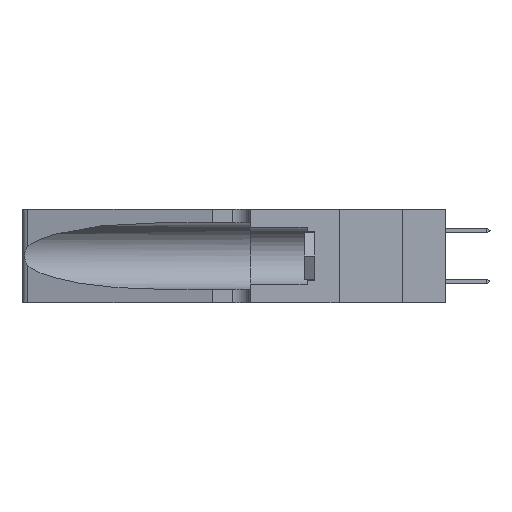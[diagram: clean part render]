
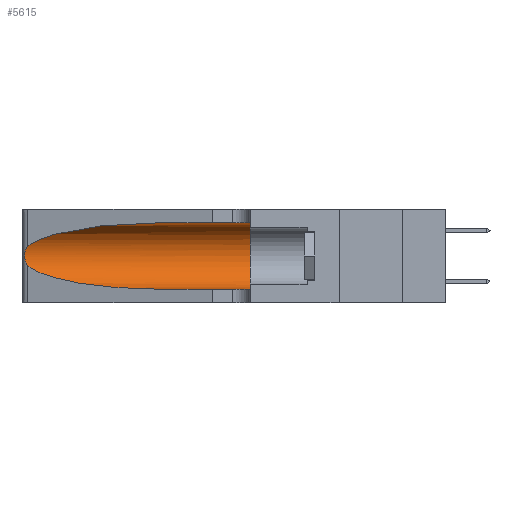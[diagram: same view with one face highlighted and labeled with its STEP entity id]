
A CAD part, left-side view. The second image highlights one B-rep face of the part: STEP entity #5615.
In plain terms, the highlighted cylindrical face has radius 3.308 mm (diameter 6.617 mm), a partial arc.
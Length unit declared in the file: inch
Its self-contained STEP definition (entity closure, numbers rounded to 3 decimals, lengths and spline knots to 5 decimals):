
#979 =( BOUNDED_CURVE ( )  B_SPLINE_CURVE ( 3, ( #26609, #16413, #6834, #9188 ),
 .UNSPECIFIED., .F., .F. ) 
 B_SPLINE_CURVE_WITH_KNOTS ( ( 4, 4 ),
 ( 3.44316, 4.71239 ),
 .UNSPECIFIED. ) 
 CURVE ( )  GEOMETRIC_REPRESENTATION_ITEM ( )  RATIONAL_B_SPLINE_CURVE ( ( 1., 0.87, 0.87, 1. ) ) 
 REPRESENTATION_ITEM ( '' )  );
#1558 = VECTOR ( 'NONE', #3697, 39.37008 ) ;
#1988 = CARTESIAN_POINT ( 'NONE',  ( 0.1305, 0.72297, 0.31525 ) ) ;
#2297 = CARTESIAN_POINT ( 'NONE',  ( 0.25854, 1.2359, 0.20912 ) ) ;
#2803 = DIRECTION ( 'NONE',  ( 0., 0., 1. ) ) ;
#3655 = DIRECTION ( 'NONE',  ( 0., -1., 0. ) ) ;
#3697 = DIRECTION ( 'NONE',  ( 0., -1., 0. ) ) ;
#3764 = CARTESIAN_POINT ( 'NONE',  ( 0.25487, 1.22718, 0.14631 ) ) ;
#3884 = CARTESIAN_POINT ( 'NONE',  ( 0.1305, 1.61858, 0.31525 ) ) ;
#3975 =( BOUNDED_CURVE ( )  B_SPLINE_CURVE ( 3, ( #1988, #10288, #7397, #22327 ),
 .UNSPECIFIED., .F., .F. ) 
 B_SPLINE_CURVE_WITH_KNOTS ( ( 4, 4 ),
 ( 1.5708, 2.84003 ),
 .UNSPECIFIED. ) 
 CURVE ( )  GEOMETRIC_REPRESENTATION_ITEM ( )  RATIONAL_B_SPLINE_CURVE ( ( 1., 0.87, 0.87, 1. ) ) 
 REPRESENTATION_ITEM ( '' )  );
#4960 = EDGE_LOOP ( 'NONE', ( #15871, #28062, #21930, #26043, #31861, #14223 ) ) ;
#5230 = CARTESIAN_POINT ( 'NONE',  ( 0.25555, 1.22994, 0.2215 ) ) ;
#5615 = ADVANCED_FACE ( 'NONE', ( #18516 ), #10312, .F. ) ;
#5752 = B_SPLINE_CURVE_WITH_KNOTS ( 'NONE', 3,
 ( #9812, #5230, #18778, #13718, #2297, #28128, #29218, #25116, #11367, #16206, #8639, #28773, #31271, #3764 ),
 .UNSPECIFIED., .F., .F.,
 ( 4, 2, 2, 2, 2, 2, 4 ),
 ( 0., 0.00027, 0.00053, 0.00107, 0.0016, 0.00187, 0.00214 ),
 .UNSPECIFIED. ) ;
#6315 = AXIS2_PLACEMENT_3D ( 'NONE', #17708, #27797, #2803 ) ;
#6834 = CARTESIAN_POINT ( 'NONE',  ( 0.18966, 0.96281, 0.05475 ) ) ;
#7397 = CARTESIAN_POINT ( 'NONE',  ( 0.2373, 1.15595, 0.28018 ) ) ;
#8072 = CIRCLE ( 'NONE', #6315, 0.13025 ) ;
#8535 = VERTEX_POINT ( 'NONE', #23528 ) ;
#8639 = CARTESIAN_POINT ( 'NONE',  ( 0.25789, 1.23486, 0.15765 ) ) ;
#8794 = CARTESIAN_POINT ( 'NONE',  ( 0.1305, 1.61858, 0.05475 ) ) ;
#9188 = CARTESIAN_POINT ( 'NONE',  ( 0.1305, 0.72297, 0.05475 ) ) ;
#9275 = CARTESIAN_POINT ( 'NONE',  ( 0.1305, 1.61858, 0.185 ) ) ;
#9812 = CARTESIAN_POINT ( 'NONE',  ( 0.25487, 1.22718, 0.22369 ) ) ;
#10288 = CARTESIAN_POINT ( 'NONE',  ( 0.18966, 0.96281, 0.31525 ) ) ;
#10312 = CYLINDRICAL_SURFACE ( 'NONE', #31719, 0.13025 ) ;
#10435 = EDGE_CURVE ( 'NONE', #23699, #16093, #979, .T. ) ;
#11166 = CARTESIAN_POINT ( 'NONE',  ( 0.1305, 0.35, 0.31525 ) ) ;
#11367 = CARTESIAN_POINT ( 'NONE',  ( 0.26017, 1.23833, 0.17102 ) ) ;
#11415 = CARTESIAN_POINT ( 'NONE',  ( 0.25487, 1.22718, 0.22369 ) ) ;
#13718 = CARTESIAN_POINT ( 'NONE',  ( 0.25787, 1.23484, 0.2124 ) ) ;
#14040 = EDGE_CURVE ( 'NONE', #26990, #23699, #5752, .T. ) ;
#14223 = ORIENTED_EDGE ( 'NONE', *, *, #25678, .F. ) ;
#15762 = CARTESIAN_POINT ( 'NONE',  ( 0.1305, 0.72297, 0.05475 ) ) ;
#15871 = ORIENTED_EDGE ( 'NONE', *, *, #27220, .T. ) ;
#16093 = VERTEX_POINT ( 'NONE', #15762 ) ;
#16206 = CARTESIAN_POINT ( 'NONE',  ( 0.25856, 1.23593, 0.16098 ) ) ;
#16413 = CARTESIAN_POINT ( 'NONE',  ( 0.2373, 1.15595, 0.08982 ) ) ;
#16650 = VERTEX_POINT ( 'NONE', #24697 ) ;
#17708 = CARTESIAN_POINT ( 'NONE',  ( 0.1305, 0.35, 0.185 ) ) ;
#18516 = FACE_OUTER_BOUND ( 'NONE', #4960, .T. ) ;
#18778 = CARTESIAN_POINT ( 'NONE',  ( 0.25639, 1.23184, 0.21858 ) ) ;
#19902 = LINE ( 'NONE', #3884, #31514 ) ;
#21930 = ORIENTED_EDGE ( 'NONE', *, *, #10435, .T. ) ;
#22327 = CARTESIAN_POINT ( 'NONE',  ( 0.25487, 1.22718, 0.22369 ) ) ;
#23528 = CARTESIAN_POINT ( 'NONE',  ( 0.1305, 0.35, 0.05475 ) ) ;
#23699 = VERTEX_POINT ( 'NONE', #31519 ) ;
#24697 = CARTESIAN_POINT ( 'NONE',  ( 0.1305, 0.72297, 0.31525 ) ) ;
#24858 = LINE ( 'NONE', #8794, #1558 ) ;
#25116 = CARTESIAN_POINT ( 'NONE',  ( 0.26075, 1.23896, 0.178 ) ) ;
#25678 = EDGE_CURVE ( 'NONE', #16650, #28597, #19902, .T. ) ;
#26043 = ORIENTED_EDGE ( 'NONE', *, *, #31710, .T. ) ;
#26609 = CARTESIAN_POINT ( 'NONE',  ( 0.25487, 1.22718, 0.14631 ) ) ;
#26696 = DIRECTION ( 'NONE',  ( 0., -1., 0. ) ) ;
#26990 = VERTEX_POINT ( 'NONE', #11415 ) ;
#27220 = EDGE_CURVE ( 'NONE', #16650, #26990, #3975, .T. ) ;
#27797 = DIRECTION ( 'NONE',  ( 0., 1., 0. ) ) ;
#28062 = ORIENTED_EDGE ( 'NONE', *, *, #14040, .T. ) ;
#28128 = CARTESIAN_POINT ( 'NONE',  ( 0.26018, 1.23835, 0.19895 ) ) ;
#28597 = VERTEX_POINT ( 'NONE', #11166 ) ;
#28773 = CARTESIAN_POINT ( 'NONE',  ( 0.25639, 1.23186, 0.15144 ) ) ;
#29218 = CARTESIAN_POINT ( 'NONE',  ( 0.26075, 1.23896, 0.19203 ) ) ;
#31271 = CARTESIAN_POINT ( 'NONE',  ( 0.25555, 1.22993, 0.14849 ) ) ;
#31514 = VECTOR ( 'NONE', #3655, 39.37008 ) ;
#31519 = CARTESIAN_POINT ( 'NONE',  ( 0.25487, 1.22718, 0.14631 ) ) ;
#31666 = DIRECTION ( 'NONE',  ( 0., 0., -1. ) ) ;
#31710 = EDGE_CURVE ( 'NONE', #16093, #8535, #24858, .T. ) ;
#31719 = AXIS2_PLACEMENT_3D ( 'NONE', #9275, #26696, #31666 ) ;
#31861 = ORIENTED_EDGE ( 'NONE', *, *, #31952, .F. ) ;
#31952 = EDGE_CURVE ( 'NONE', #28597, #8535, #8072, .T. ) ;
